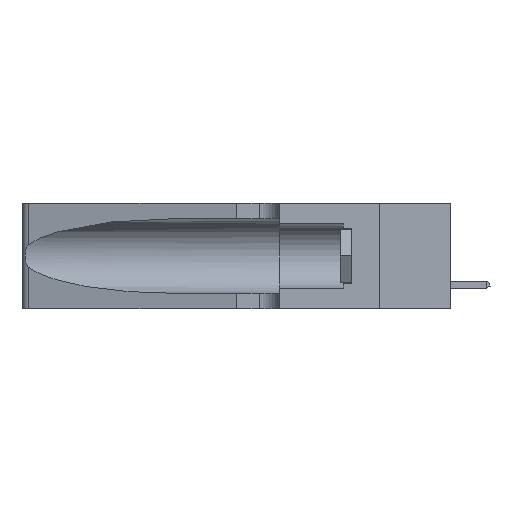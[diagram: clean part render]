
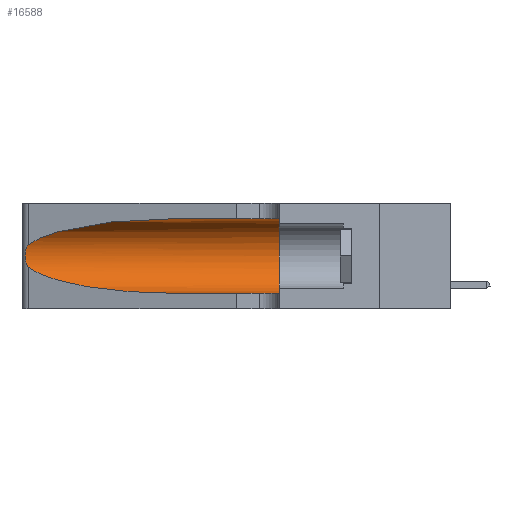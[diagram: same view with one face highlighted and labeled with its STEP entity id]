
A CAD part, left-side view. The second image highlights one B-rep face of the part: STEP entity #16588.
In plain terms, the highlighted cylindrical face has radius 3.308 mm (diameter 6.617 mm), a partial arc.
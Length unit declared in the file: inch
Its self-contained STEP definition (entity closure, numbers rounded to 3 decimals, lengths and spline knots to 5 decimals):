
#1096 = CARTESIAN_POINT ( 'NONE',  ( 0.25487, 1.22718, 0.14631 ) ) ;
#1263 = LINE ( 'NONE', #24942, #22586 ) ;
#1940 = CARTESIAN_POINT ( 'NONE',  ( 0.1305, 1.61858, 0.31525 ) ) ;
#2592 = ORIENTED_EDGE ( 'NONE', *, *, #44428, .T. ) ;
#3082 = CARTESIAN_POINT ( 'NONE',  ( 0.1305, 0.72297, 0.05475 ) ) ;
#5014 = CARTESIAN_POINT ( 'NONE',  ( 0.25487, 1.22718, 0.22369 ) ) ;
#5174 = CARTESIAN_POINT ( 'NONE',  ( 0.25854, 1.2359, 0.20912 ) ) ;
#6518 = CARTESIAN_POINT ( 'NONE',  ( 0.2373, 1.15595, 0.08982 ) ) ;
#6868 = CARTESIAN_POINT ( 'NONE',  ( 0.25487, 1.22718, 0.14631 ) ) ;
#6968 = CARTESIAN_POINT ( 'NONE',  ( 0.1305, 0.72297, 0.31525 ) ) ;
#7652 = AXIS2_PLACEMENT_3D ( 'NONE', #32614, #48269, #40270 ) ;
#8416 = EDGE_CURVE ( 'NONE', #38120, #38496, #20037, .T. ) ;
#9696 = CARTESIAN_POINT ( 'NONE',  ( 0.1305, 0.72297, 0.05475 ) ) ;
#11162 = DIRECTION ( 'NONE',  ( 0., -1., 0. ) ) ;
#13818 = CARTESIAN_POINT ( 'NONE',  ( 0.25639, 1.23186, 0.15144 ) ) ;
#13999 = CARTESIAN_POINT ( 'NONE',  ( 0.25487, 1.22718, 0.14631 ) ) ;
#14329 = EDGE_CURVE ( 'NONE', #25683, #40507, #33419, .T. ) ;
#15220 = DIRECTION ( 'NONE',  ( 0., 0., -1. ) ) ;
#15780 = ORIENTED_EDGE ( 'NONE', *, *, #14329, .T. ) ;
#16564 = CARTESIAN_POINT ( 'NONE',  ( 0.26075, 1.23896, 0.178 ) ) ;
#16588 = ADVANCED_FACE ( 'NONE', ( #49058 ), #31436, .F. ) ;
#16706 = CARTESIAN_POINT ( 'NONE',  ( 0.1305, 0.35, 0.05475 ) ) ;
#18135 = CARTESIAN_POINT ( 'NONE',  ( 0.18966, 0.96281, 0.31525 ) ) ;
#20037 = LINE ( 'NONE', #1940, #38336 ) ;
#21142 = CARTESIAN_POINT ( 'NONE',  ( 0.26018, 1.23835, 0.19895 ) ) ;
#21912 = CARTESIAN_POINT ( 'NONE',  ( 0.2373, 1.15595, 0.28018 ) ) ;
#21997 = CARTESIAN_POINT ( 'NONE',  ( 0.25856, 1.23593, 0.16098 ) ) ;
#22569 = CARTESIAN_POINT ( 'NONE',  ( 0.1305, 1.61858, 0.185 ) ) ;
#22586 = VECTOR ( 'NONE', #47937, 39.37008 ) ;
#23049 = EDGE_LOOP ( 'NONE', ( #48251, #25172, #15780, #2592, #33139, #29541 ) ) ;
#23395 = EDGE_CURVE ( 'NONE', #42056, #25683, #45486, .T. ) ;
#24942 = CARTESIAN_POINT ( 'NONE',  ( 0.1305, 1.61858, 0.05475 ) ) ;
#25172 = ORIENTED_EDGE ( 'NONE', *, *, #23395, .T. ) ;
#25683 = VERTEX_POINT ( 'NONE', #1096 ) ;
#28087 = VERTEX_POINT ( 'NONE', #16706 ) ;
#28439 = AXIS2_PLACEMENT_3D ( 'NONE', #22569, #11162, #15220 ) ;
#28982 =( BOUNDED_CURVE ( )  B_SPLINE_CURVE ( 3, ( #6968, #18135, #21912, #45399 ),
 .UNSPECIFIED., .F., .F. ) 
 B_SPLINE_CURVE_WITH_KNOTS ( ( 4, 4 ),
 ( 1.5708, 2.84003 ),
 .UNSPECIFIED. ) 
 CURVE ( )  GEOMETRIC_REPRESENTATION_ITEM ( )  RATIONAL_B_SPLINE_CURVE ( ( 1., 0.87, 0.87, 1. ) ) 
 REPRESENTATION_ITEM ( '' )  );
#29541 = ORIENTED_EDGE ( 'NONE', *, *, #8416, .F. ) ;
#31436 = CYLINDRICAL_SURFACE ( 'NONE', #28439, 0.13025 ) ;
#32614 = CARTESIAN_POINT ( 'NONE',  ( 0.1305, 0.35, 0.185 ) ) ;
#33122 = DIRECTION ( 'NONE',  ( 0., -1., 0. ) ) ;
#33139 = ORIENTED_EDGE ( 'NONE', *, *, #44326, .F. ) ;
#33419 =( BOUNDED_CURVE ( )  B_SPLINE_CURVE ( 3, ( #6868, #6518, #41563, #3082 ),
 .UNSPECIFIED., .F., .F. ) 
 B_SPLINE_CURVE_WITH_KNOTS ( ( 4, 4 ),
 ( 3.44316, 4.71239 ),
 .UNSPECIFIED. ) 
 CURVE ( )  GEOMETRIC_REPRESENTATION_ITEM ( )  RATIONAL_B_SPLINE_CURVE ( ( 1., 0.87, 0.87, 1. ) ) 
 REPRESENTATION_ITEM ( '' )  );
#34102 = CARTESIAN_POINT ( 'NONE',  ( 0.1305, 0.72297, 0.31525 ) ) ;
#34175 = CIRCLE ( 'NONE', #7652, 0.13025 ) ;
#35977 = CARTESIAN_POINT ( 'NONE',  ( 0.26075, 1.23896, 0.19203 ) ) ;
#36317 = CARTESIAN_POINT ( 'NONE',  ( 0.25787, 1.23484, 0.2124 ) ) ;
#36639 = EDGE_CURVE ( 'NONE', #38120, #42056, #28982, .T. ) ;
#36648 = CARTESIAN_POINT ( 'NONE',  ( 0.25555, 1.22994, 0.2215 ) ) ;
#38120 = VERTEX_POINT ( 'NONE', #34102 ) ;
#38336 = VECTOR ( 'NONE', #33122, 39.37008 ) ;
#38496 = VERTEX_POINT ( 'NONE', #45278 ) ;
#40270 = DIRECTION ( 'NONE',  ( 0., 0., 1. ) ) ;
#40507 = VERTEX_POINT ( 'NONE', #9696 ) ;
#40727 = CARTESIAN_POINT ( 'NONE',  ( 0.25789, 1.23486, 0.15765 ) ) ;
#41563 = CARTESIAN_POINT ( 'NONE',  ( 0.18966, 0.96281, 0.05475 ) ) ;
#42056 = VERTEX_POINT ( 'NONE', #46655 ) ;
#44326 = EDGE_CURVE ( 'NONE', #38496, #28087, #34175, .T. ) ;
#44428 = EDGE_CURVE ( 'NONE', #40507, #28087, #1263, .T. ) ;
#45278 = CARTESIAN_POINT ( 'NONE',  ( 0.1305, 0.35, 0.31525 ) ) ;
#45306 = CARTESIAN_POINT ( 'NONE',  ( 0.25555, 1.22993, 0.14849 ) ) ;
#45399 = CARTESIAN_POINT ( 'NONE',  ( 0.25487, 1.22718, 0.22369 ) ) ;
#45486 = B_SPLINE_CURVE_WITH_KNOTS ( 'NONE', 3,
 ( #5014, #36648, #47726, #36317, #5174, #21142, #35977, #16564, #48560, #21997, #40727, #13818, #45306, #13999 ),
 .UNSPECIFIED., .F., .F.,
 ( 4, 2, 2, 2, 2, 2, 4 ),
 ( 0., 0.00027, 0.00053, 0.00107, 0.0016, 0.00187, 0.00214 ),
 .UNSPECIFIED. ) ;
#46655 = CARTESIAN_POINT ( 'NONE',  ( 0.25487, 1.22718, 0.22369 ) ) ;
#47726 = CARTESIAN_POINT ( 'NONE',  ( 0.25639, 1.23184, 0.21858 ) ) ;
#47937 = DIRECTION ( 'NONE',  ( 0., -1., 0. ) ) ;
#48251 = ORIENTED_EDGE ( 'NONE', *, *, #36639, .T. ) ;
#48269 = DIRECTION ( 'NONE',  ( 0., 1., 0. ) ) ;
#48560 = CARTESIAN_POINT ( 'NONE',  ( 0.26017, 1.23833, 0.17102 ) ) ;
#49058 = FACE_OUTER_BOUND ( 'NONE', #23049, .T. ) ;
